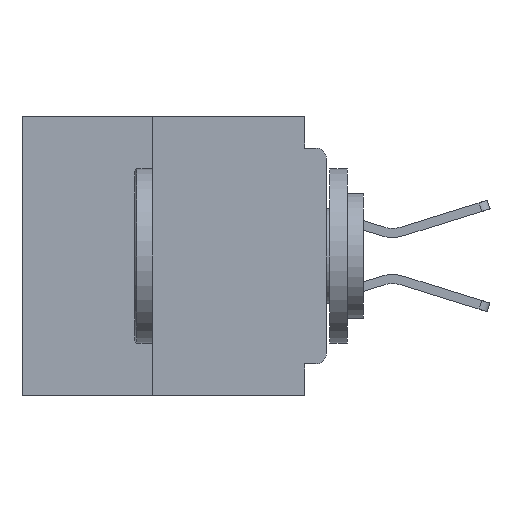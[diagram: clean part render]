
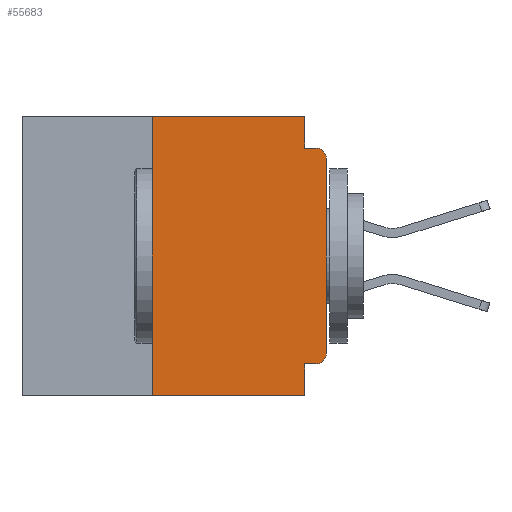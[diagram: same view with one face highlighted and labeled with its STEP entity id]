
A CAD part, left-side view. The second image highlights one B-rep face of the part: STEP entity #55683.
In plain terms, the highlighted planar face has unit normal (-1, 0, 0).
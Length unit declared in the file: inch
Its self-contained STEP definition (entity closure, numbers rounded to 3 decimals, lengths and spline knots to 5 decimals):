
#592 = VECTOR ( 'NONE', #7319, 39.37008 ) ;
#616 = CARTESIAN_POINT ( 'NONE',  ( 0., 0., -0.06 ) ) ;
#3558 = CARTESIAN_POINT ( 'NONE',  ( 0., 0.437, 0. ) ) ;
#3963 = EDGE_CURVE ( 'NONE', #17474, #57155, #47555, .T. ) ;
#4094 = VERTEX_POINT ( 'NONE', #16977 ) ;
#5114 = DIRECTION ( 'NONE',  ( 1., 0., 0. ) ) ;
#5541 = LINE ( 'NONE', #28395, #23632 ) ;
#5862 = EDGE_CURVE ( 'NONE', #4094, #52364, #18327, .T. ) ;
#5981 = ORIENTED_EDGE ( 'NONE', *, *, #34887, .F. ) ;
#7132 = CARTESIAN_POINT ( 'NONE',  ( 0., 0.25, -0.4 ) ) ;
#7319 = DIRECTION ( 'NONE',  ( 0., 0., 1. ) ) ;
#8078 = CARTESIAN_POINT ( 'NONE',  ( 0., 0.015, -0.355 ) ) ;
#8454 = DIRECTION ( 'NONE',  ( 0., -1., 0. ) ) ;
#9243 = CARTESIAN_POINT ( 'NONE',  ( 0., 0.031, 0. ) ) ;
#9278 = ORIENTED_EDGE ( 'NONE', *, *, #5862, .F. ) ;
#9857 = EDGE_CURVE ( 'NONE', #57155, #4094, #35230, .T. ) ;
#10152 = DIRECTION ( 'NONE',  ( -1., 0., 0. ) ) ;
#10753 = VERTEX_POINT ( 'NONE', #44951 ) ;
#11967 = CARTESIAN_POINT ( 'NONE',  ( 0., 0.031, -0.4 ) ) ;
#12975 = VECTOR ( 'NONE', #34676, 39.37008 ) ;
#13798 = VERTEX_POINT ( 'NONE', #8078 ) ;
#14458 = VERTEX_POINT ( 'NONE', #21463 ) ;
#14549 = VERTEX_POINT ( 'NONE', #44219 ) ;
#15114 = EDGE_CURVE ( 'NONE', #52364, #14549, #31015, .T. ) ;
#15215 = ORIENTED_EDGE ( 'NONE', *, *, #34810, .T. ) ;
#15808 = ORIENTED_EDGE ( 'NONE', *, *, #15114, .F. ) ;
#16977 = CARTESIAN_POINT ( 'NONE',  ( 0., 0.031, 0. ) ) ;
#17474 = VERTEX_POINT ( 'NONE', #7132 ) ;
#17538 = LINE ( 'NONE', #35078, #29329 ) ;
#18327 = LINE ( 'NONE', #9243, #52162 ) ;
#19390 = ORIENTED_EDGE ( 'NONE', *, *, #9857, .F. ) ;
#19694 = DIRECTION ( 'NONE',  ( -1., 0., 0. ) ) ;
#20913 = VERTEX_POINT ( 'NONE', #33597 ) ;
#21463 = CARTESIAN_POINT ( 'NONE',  ( 0., 0.031, -0.355 ) ) ;
#22844 = EDGE_CURVE ( 'NONE', #46214, #14549, #27600, .T. ) ;
#23632 = VECTOR ( 'NONE', #32850, 39.37008 ) ;
#25408 = ORIENTED_EDGE ( 'NONE', *, *, #56456, .T. ) ;
#25418 = DIRECTION ( 'NONE',  ( 0., 0., -1. ) ) ;
#25503 = ORIENTED_EDGE ( 'NONE', *, *, #56457, .F. ) ;
#26041 = AXIS2_PLACEMENT_3D ( 'NONE', #46121, #19694, #50531 ) ;
#27369 = CARTESIAN_POINT ( 'NONE',  ( 0., 0.25, 0. ) ) ;
#27600 = CIRCLE ( 'NONE', #37968, 0.015 ) ;
#28259 = VECTOR ( 'NONE', #39169, 39.37008 ) ;
#28395 = CARTESIAN_POINT ( 'NONE',  ( 0., 0., -0.355 ) ) ;
#29329 = VECTOR ( 'NONE', #8454, 39.37008 ) ;
#29483 = CARTESIAN_POINT ( 'NONE',  ( 0., 0., 0. ) ) ;
#31015 = LINE ( 'NONE', #34753, #28259 ) ;
#31752 = CARTESIAN_POINT ( 'NONE',  ( 0., 0.437, 0. ) ) ;
#32850 = DIRECTION ( 'NONE',  ( 0., 1., 0. ) ) ;
#33372 = CARTESIAN_POINT ( 'NONE',  ( 0., 0.031, -0.045 ) ) ;
#33597 = CARTESIAN_POINT ( 'NONE',  ( 0., 0., -0.34 ) ) ;
#34676 = DIRECTION ( 'NONE',  ( 0., -1., 0. ) ) ;
#34753 = CARTESIAN_POINT ( 'NONE',  ( 0., 0., -0.045 ) ) ;
#34810 = EDGE_CURVE ( 'NONE', #20913, #46214, #37504, .T. ) ;
#34887 = EDGE_CURVE ( 'NONE', #14458, #10753, #55383, .T. ) ;
#35067 = ORIENTED_EDGE ( 'NONE', *, *, #3963, .F. ) ;
#35078 = CARTESIAN_POINT ( 'NONE',  ( 0., 0.437, -0.4 ) ) ;
#35230 = LINE ( 'NONE', #3558, #12975 ) ;
#36203 = DIRECTION ( 'NONE',  ( 0., 0., -1. ) ) ;
#36756 = CARTESIAN_POINT ( 'NONE',  ( 0., 0.015, -0.06 ) ) ;
#37256 = VECTOR ( 'NONE', #55227, 39.37008 ) ;
#37504 = LINE ( 'NONE', #29483, #592 ) ;
#37968 = AXIS2_PLACEMENT_3D ( 'NONE', #36756, #10152, #41162 ) ;
#38251 = ORIENTED_EDGE ( 'NONE', *, *, #22844, .T. ) ;
#39169 = DIRECTION ( 'NONE',  ( 0., -1., 0. ) ) ;
#41162 = DIRECTION ( 'NONE',  ( 0., 0., -1. ) ) ;
#43664 = VECTOR ( 'NONE', #25418, 39.37008 ) ;
#44219 = CARTESIAN_POINT ( 'NONE',  ( 0., 0.015, -0.045 ) ) ;
#44691 = DIRECTION ( 'NONE',  ( 0., 0., -1. ) ) ;
#44951 = CARTESIAN_POINT ( 'NONE',  ( 0., 0.031, -0.4 ) ) ;
#46121 = CARTESIAN_POINT ( 'NONE',  ( 0., 0.015, -0.34 ) ) ;
#46214 = VERTEX_POINT ( 'NONE', #616 ) ;
#47119 = CIRCLE ( 'NONE', #26041, 0.015 ) ;
#47555 = LINE ( 'NONE', #55339, #37256 ) ;
#49999 = AXIS2_PLACEMENT_3D ( 'NONE', #31752, #5114, #36203 ) ;
#50531 = DIRECTION ( 'NONE',  ( 0., 0., -1. ) ) ;
#51103 = ORIENTED_EDGE ( 'NONE', *, *, #55531, .T. ) ;
#52162 = VECTOR ( 'NONE', #44691, 39.37008 ) ;
#52364 = VERTEX_POINT ( 'NONE', #33372 ) ;
#53708 = PLANE ( 'NONE',  #49999 ) ;
#54780 = EDGE_LOOP ( 'NONE', ( #15215, #38251, #15808, #9278, #19390, #35067, #51103, #5981, #25503, #25408 ) ) ;
#55227 = DIRECTION ( 'NONE',  ( 0., 0., 1. ) ) ;
#55339 = CARTESIAN_POINT ( 'NONE',  ( 0., 0.25, -0.4 ) ) ;
#55383 = LINE ( 'NONE', #11967, #43664 ) ;
#55531 = EDGE_CURVE ( 'NONE', #17474, #10753, #17538, .T. ) ;
#55683 = ADVANCED_FACE ( 'NONE', ( #57439 ), #53708, .F. ) ;
#56456 = EDGE_CURVE ( 'NONE', #13798, #20913, #47119, .T. ) ;
#56457 = EDGE_CURVE ( 'NONE', #13798, #14458, #5541, .T. ) ;
#57155 = VERTEX_POINT ( 'NONE', #27369 ) ;
#57439 = FACE_OUTER_BOUND ( 'NONE', #54780, .T. ) ;
